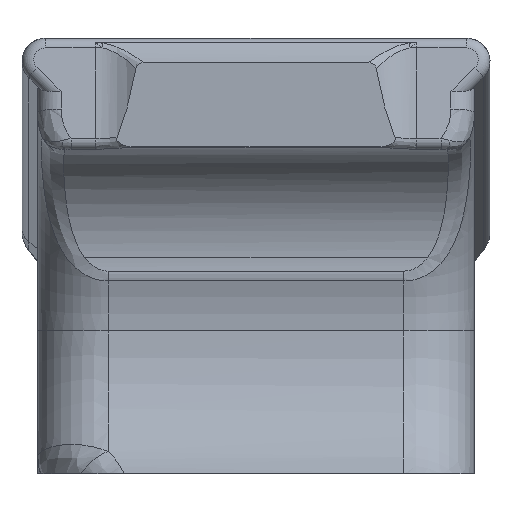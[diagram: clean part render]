
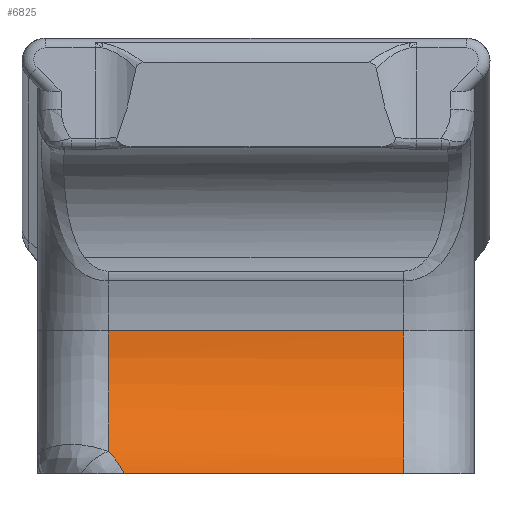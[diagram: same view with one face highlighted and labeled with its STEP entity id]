
A CAD part, left-side view. The second image highlights one B-rep face of the part: STEP entity #6825.
In plain terms, the highlighted cylindrical face has radius 14.287 mm (diameter 28.575 mm), a partial arc.
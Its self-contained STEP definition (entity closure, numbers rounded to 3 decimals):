
#151 = CARTESIAN_POINT ( 'NONE',  ( 90.94, -44.575, -0.458 ) ) ;
#437 = CYLINDRICAL_SURFACE ( 'NONE', #4892, 14.288 ) ;
#718 = B_SPLINE_CURVE_WITH_KNOTS ( 'NONE', 3,
 ( #3565, #10119, #1736, #6350, #7233, #6504, #6581, #2602, #4145, #2440, #2365, #1560, #10167, #10071 ),
 .UNSPECIFIED., .F., .F.,
 ( 4, 2, 2, 1, 1, 2, 2, 4 ),
 ( 0., 0.25, 0.375, 0.437, 0.469, 0.484, 0.5, 1. ),
 .UNSPECIFIED. ) ;
#768 = LINE ( 'NONE', #7732, #5046 ) ;
#1304 = DIRECTION ( 'NONE',  ( 0., 1., 0. ) ) ;
#1312 = VECTOR ( 'NONE', #9054, 1000. ) ;
#1504 = CARTESIAN_POINT ( 'NONE',  ( 86.612, -44.575, -10.701 ) ) ;
#1560 = CARTESIAN_POINT ( 'NONE',  ( 85.113, -45.624, -11.981 ) ) ;
#1736 = CARTESIAN_POINT ( 'NONE',  ( 86.281, -44.89, -11.016 ) ) ;
#2031 = CARTESIAN_POINT ( 'NONE',  ( 84.171, -69.708, -12.607 ) ) ;
#2339 = VERTEX_POINT ( 'NONE', #2031 ) ;
#2365 = CARTESIAN_POINT ( 'NONE',  ( 85.515, -45.405, -11.664 ) ) ;
#2440 = CARTESIAN_POINT ( 'NONE',  ( 85.529, -45.397, -11.653 ) ) ;
#2587 = ORIENTED_EDGE ( 'NONE', *, *, #8551, .T. ) ;
#2602 = CARTESIAN_POINT ( 'NONE',  ( 85.595, -45.361, -11.601 ) ) ;
#2708 = VERTEX_POINT ( 'NONE', #151 ) ;
#2800 = CARTESIAN_POINT ( 'NONE',  ( 76.653, -44.575, -0.458 ) ) ;
#2917 = CARTESIAN_POINT ( 'NONE',  ( 76.653, -69.708, -0.458 ) ) ;
#2922 = EDGE_CURVE ( 'NONE', #8086, #9967, #718, .T. ) ;
#3543 = VERTEX_POINT ( 'NONE', #5366 ) ;
#3565 = CARTESIAN_POINT ( 'NONE',  ( 86.612, -44.575, -10.701 ) ) ;
#3654 = DIRECTION ( 'NONE',  ( 1., 0., 0. ) ) ;
#3777 = DIRECTION ( 'NONE',  ( 1., 0., 0. ) ) ;
#3842 = AXIS2_PLACEMENT_3D ( 'NONE', #2800, #8207, #3654 ) ;
#3864 = ORIENTED_EDGE ( 'NONE', *, *, #2922, .T. ) ;
#3907 = CARTESIAN_POINT ( 'NONE',  ( 76.653, -71.429, -0.458 ) ) ;
#3952 = DIRECTION ( 'NONE',  ( 0., -1., 0. ) ) ;
#4145 = CARTESIAN_POINT ( 'NONE',  ( 85.556, -45.383, -11.632 ) ) ;
#4176 = CIRCLE ( 'NONE', #3842, 14.288 ) ;
#4647 = CARTESIAN_POINT ( 'NONE',  ( 90.94, -71.429, -0.458 ) ) ;
#4892 = AXIS2_PLACEMENT_3D ( 'NONE', #3907, #1304, #9852 ) ;
#5046 = VECTOR ( 'NONE', #3952, 1000. ) ;
#5366 = CARTESIAN_POINT ( 'NONE',  ( 90.94, -69.708, -0.458 ) ) ;
#5495 = ORIENTED_EDGE ( 'NONE', *, *, #9636, .T. ) ;
#5607 = ORIENTED_EDGE ( 'NONE', *, *, #9493, .T. ) ;
#6023 = CIRCLE ( 'NONE', #9759, 14.288 ) ;
#6350 = CARTESIAN_POINT ( 'NONE',  ( 86.004, -45.099, -11.26 ) ) ;
#6423 = CARTESIAN_POINT ( 'NONE',  ( 84.171, -45.933, -12.607 ) ) ;
#6504 = CARTESIAN_POINT ( 'NONE',  ( 85.761, -45.261, -11.466 ) ) ;
#6581 = CARTESIAN_POINT ( 'NONE',  ( 85.685, -45.308, -11.528 ) ) ;
#6825 = ADVANCED_FACE ( 'NONE', ( #7015 ), #437, .F. ) ;
#7015 = FACE_OUTER_BOUND ( 'NONE', #9349, .T. ) ;
#7074 = ORIENTED_EDGE ( 'NONE', *, *, #9773, .T. ) ;
#7233 = CARTESIAN_POINT ( 'NONE',  ( 85.909, -45.166, -11.342 ) ) ;
#7732 = CARTESIAN_POINT ( 'NONE',  ( 84.171, -71.429, -12.607 ) ) ;
#8086 = VERTEX_POINT ( 'NONE', #1504 ) ;
#8207 = DIRECTION ( 'NONE',  ( 0., 1., 0. ) ) ;
#8320 = DIRECTION ( 'NONE',  ( 0., -1., 0. ) ) ;
#8551 = EDGE_CURVE ( 'NONE', #2339, #3543, #6023, .T. ) ;
#9054 = DIRECTION ( 'NONE',  ( 0., 1., 0. ) ) ;
#9349 = EDGE_LOOP ( 'NONE', ( #2587, #5495, #5607, #3864, #7074 ) ) ;
#9493 = EDGE_CURVE ( 'NONE', #2708, #8086, #4176, .T. ) ;
#9604 = LINE ( 'NONE', #4647, #1312 ) ;
#9636 = EDGE_CURVE ( 'NONE', #3543, #2708, #9604, .T. ) ;
#9759 = AXIS2_PLACEMENT_3D ( 'NONE', #2917, #8320, #3777 ) ;
#9773 = EDGE_CURVE ( 'NONE', #9967, #2339, #768, .T. ) ;
#9852 = DIRECTION ( 'NONE',  ( 1., 0., 0. ) ) ;
#9967 = VERTEX_POINT ( 'NONE', #6423 ) ;
#10071 = CARTESIAN_POINT ( 'NONE',  ( 84.171, -45.933, -12.607 ) ) ;
#10119 = CARTESIAN_POINT ( 'NONE',  ( 86.453, -44.738, -10.856 ) ) ;
#10167 = CARTESIAN_POINT ( 'NONE',  ( 84.671, -45.798, -12.297 ) ) ;
